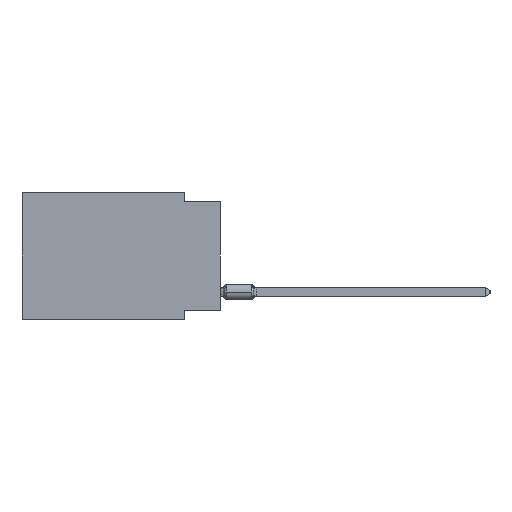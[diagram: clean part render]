
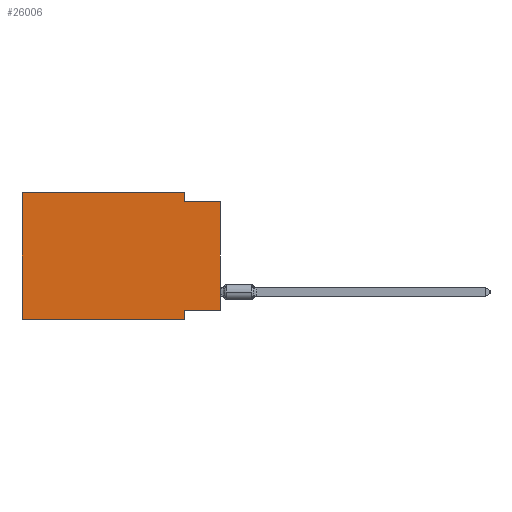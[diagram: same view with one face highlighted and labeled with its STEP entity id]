
A CAD part, left-side view. The second image highlights one B-rep face of the part: STEP entity #26006.
In plain terms, the highlighted planar face has unit normal (-1, 0, 0).
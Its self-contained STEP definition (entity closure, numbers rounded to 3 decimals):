
#2336 = ORIENTED_EDGE ( 'NONE', *, *, #24549, .F. ) ;
#2912 = DIRECTION ( 'NONE',  ( 0., -1., 0. ) ) ;
#3009 = CARTESIAN_POINT ( 'NONE',  ( 0., 13.97, -8.89 ) ) ;
#3639 = EDGE_CURVE ( 'NONE', #45698, #59790, #59156, .T. ) ;
#5307 = CARTESIAN_POINT ( 'NONE',  ( 0., 0., -0.635 ) ) ;
#5522 = LINE ( 'NONE', #29024, #60782 ) ;
#6034 = DIRECTION ( 'NONE',  ( 0., 1., 0. ) ) ;
#6134 = ORIENTED_EDGE ( 'NONE', *, *, #12238, .F. ) ;
#6765 = EDGE_CURVE ( 'NONE', #18992, #7341, #51388, .T. ) ;
#6921 = CARTESIAN_POINT ( 'NONE',  ( 0., 0., -8.255 ) ) ;
#7341 = VERTEX_POINT ( 'NONE', #34963 ) ;
#10312 = LINE ( 'NONE', #29684, #49125 ) ;
#11555 = PLANE ( 'NONE',  #16718 ) ;
#12238 = EDGE_CURVE ( 'NONE', #14560, #34840, #62107, .T. ) ;
#12992 = ORIENTED_EDGE ( 'NONE', *, *, #42221, .F. ) ;
#13106 = CARTESIAN_POINT ( 'NONE',  ( 0., 2.54, 0. ) ) ;
#13135 = VERTEX_POINT ( 'NONE', #5307 ) ;
#13982 = ORIENTED_EDGE ( 'NONE', *, *, #55374, .F. ) ;
#14560 = VERTEX_POINT ( 'NONE', #16480 ) ;
#15042 = DIRECTION ( 'NONE',  ( 0., 0., -1. ) ) ;
#16480 = CARTESIAN_POINT ( 'NONE',  ( 0., 2.54, 0. ) ) ;
#16718 = AXIS2_PLACEMENT_3D ( 'NONE', #40200, #30312, #59918 ) ;
#18992 = VERTEX_POINT ( 'NONE', #40749 ) ;
#20426 = LINE ( 'NONE', #24548, #54226 ) ;
#24130 = CARTESIAN_POINT ( 'NONE',  ( 0., 0., -0.635 ) ) ;
#24548 = CARTESIAN_POINT ( 'NONE',  ( 0., 0., 0. ) ) ;
#24549 = EDGE_CURVE ( 'NONE', #18992, #38198, #10312, .T. ) ;
#24713 = VECTOR ( 'NONE', #2912, 1000. ) ;
#24758 = LINE ( 'NONE', #24130, #45913 ) ;
#25518 = FACE_OUTER_BOUND ( 'NONE', #45379, .T. ) ;
#26006 = ADVANCED_FACE ( 'NONE', ( #25518 ), #11555, .F. ) ;
#27385 = DIRECTION ( 'NONE',  ( 0., 0., 1. ) ) ;
#29024 = CARTESIAN_POINT ( 'NONE',  ( 0., 2.54, -8.89 ) ) ;
#29454 = VECTOR ( 'NONE', #32509, 1000. ) ;
#29684 = CARTESIAN_POINT ( 'NONE',  ( 0., 13.97, 0. ) ) ;
#30312 = DIRECTION ( 'NONE',  ( 1., 0., 0. ) ) ;
#31527 = ORIENTED_EDGE ( 'NONE', *, *, #3639, .F. ) ;
#32509 = DIRECTION ( 'NONE',  ( 0., 0., -1. ) ) ;
#34048 = CARTESIAN_POINT ( 'NONE',  ( 0., 2.54, -0.635 ) ) ;
#34840 = VERTEX_POINT ( 'NONE', #34048 ) ;
#34963 = CARTESIAN_POINT ( 'NONE',  ( 0., 2.54, -8.89 ) ) ;
#35241 = ORIENTED_EDGE ( 'NONE', *, *, #58315, .T. ) ;
#37779 = ORIENTED_EDGE ( 'NONE', *, *, #6765, .T. ) ;
#38198 = VERTEX_POINT ( 'NONE', #44253 ) ;
#39848 = DIRECTION ( 'NONE',  ( 0., 0., 1. ) ) ;
#40200 = CARTESIAN_POINT ( 'NONE',  ( 0., 13.97, 0. ) ) ;
#40749 = CARTESIAN_POINT ( 'NONE',  ( 0., 13.97, -8.89 ) ) ;
#41238 = ORIENTED_EDGE ( 'NONE', *, *, #46301, .F. ) ;
#42221 = EDGE_CURVE ( 'NONE', #59790, #7341, #5522, .T. ) ;
#42462 = DIRECTION ( 'NONE',  ( 0., -1., 0. ) ) ;
#44253 = CARTESIAN_POINT ( 'NONE',  ( 0., 13.97, 0. ) ) ;
#45379 = EDGE_LOOP ( 'NONE', ( #35241, #41238, #6134, #13982, #2336, #37779, #12992, #31527 ) ) ;
#45698 = VERTEX_POINT ( 'NONE', #6921 ) ;
#45913 = VECTOR ( 'NONE', #57888, 1000. ) ;
#46301 = EDGE_CURVE ( 'NONE', #34840, #13135, #24758, .T. ) ;
#46517 = CARTESIAN_POINT ( 'NONE',  ( 0., 13.97, 0. ) ) ;
#49125 = VECTOR ( 'NONE', #27385, 1000. ) ;
#49618 = CARTESIAN_POINT ( 'NONE',  ( 0., 0., -8.255 ) ) ;
#50280 = CARTESIAN_POINT ( 'NONE',  ( 0., 2.54, -8.255 ) ) ;
#51388 = LINE ( 'NONE', #3009, #53299 ) ;
#53299 = VECTOR ( 'NONE', #42462, 1000. ) ;
#54226 = VECTOR ( 'NONE', #39848, 1000. ) ;
#55374 = EDGE_CURVE ( 'NONE', #38198, #14560, #61154, .T. ) ;
#57208 = VECTOR ( 'NONE', #6034, 1000. ) ;
#57888 = DIRECTION ( 'NONE',  ( 0., -1., 0. ) ) ;
#58315 = EDGE_CURVE ( 'NONE', #45698, #13135, #20426, .T. ) ;
#59156 = LINE ( 'NONE', #49618, #57208 ) ;
#59790 = VERTEX_POINT ( 'NONE', #50280 ) ;
#59918 = DIRECTION ( 'NONE',  ( 0., 0., -1. ) ) ;
#60782 = VECTOR ( 'NONE', #15042, 1000. ) ;
#61154 = LINE ( 'NONE', #46517, #24713 ) ;
#62107 = LINE ( 'NONE', #13106, #29454 ) ;
